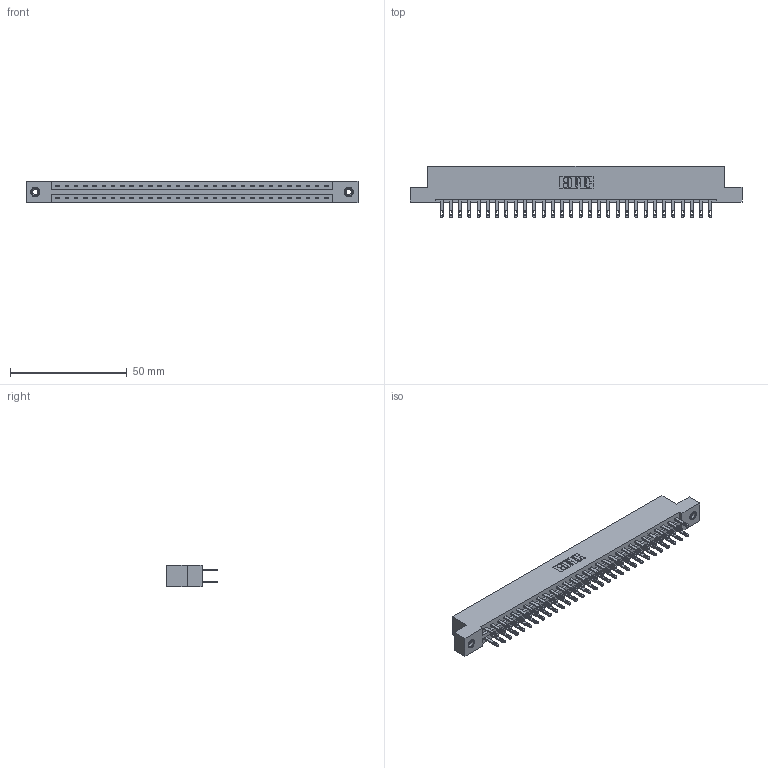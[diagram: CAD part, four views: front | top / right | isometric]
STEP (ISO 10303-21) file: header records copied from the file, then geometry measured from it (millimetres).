
FILE_DESCRIPTION (( 'STEP AP203' ), '1' );
FILE_NAME ('337-060-500-208.STEP', '2018-08-10T06:50:35', ( '' ), ( '' ), 'SwSTEP 2.0', 'SolidWorks 2016', '' );
FILE_SCHEMA (( 'CONFIG_CONTROL_DESIGN' ));
Length unit declared in the file: inch
Products named in the file (4): 337 Part_Flush Mounting Lugs - 0.156 Dia-TI; 345-292-001_345-293-100; 345-250-001_345-250-003-102; 337-060-500-208
Assembly tree (63 placements, depth 2):
  337-060-500-208
    337 Part_Flush Mounting Lugs - 0.156 Dia-TI
    345-292-001_345-293-100  x60
    345-250-001_345-250-003-102  x2
Bounding box: 141.88 x 21.85 x 9.4 mm (x, y, z)
Volume: 14970 mm3; surface area: 17496.7 mm2
Topology: 63 solids, 63 shells, 3174 faces, 9627 edges, 6410 vertices
Faces by surface type: plane 2022, cylinder 1136, cone 12, torus 4
Entity records: 25928 total; most frequent: CARTESIAN_POINT 4357, ORIENTED_EDGE 4286, DIRECTION 3761, EDGE_CURVE 2143, VECTOR 1991, LINE 1991, VERTEX_POINT 1424, AXIS2_PLACEMENT_3D 885
